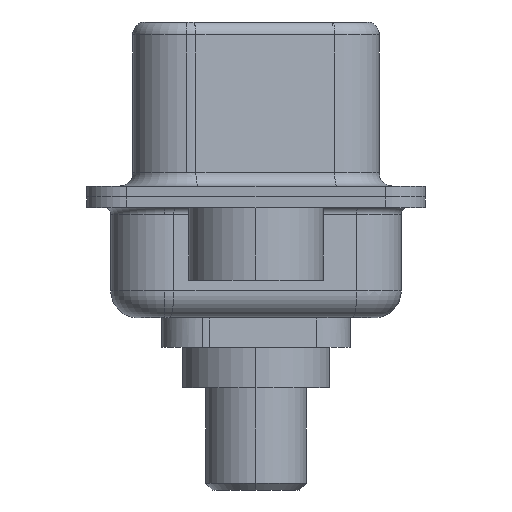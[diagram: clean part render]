
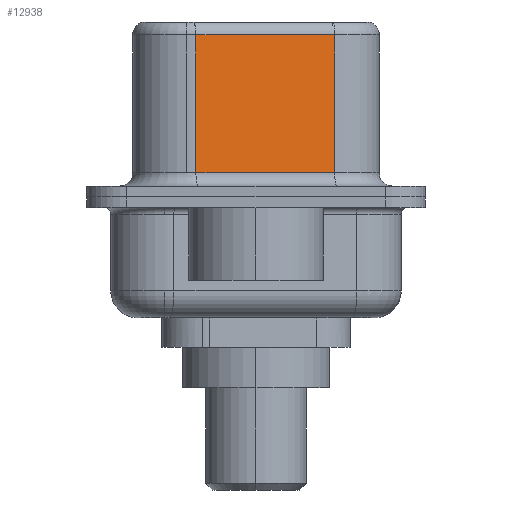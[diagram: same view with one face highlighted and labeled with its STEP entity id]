
A CAD part, left-side view. The second image highlights one B-rep face of the part: STEP entity #12938.
In plain terms, the highlighted planar face has unit normal (-0.985, -0.174, 0).
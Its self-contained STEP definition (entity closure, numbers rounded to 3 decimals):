
#333 = LINE ( 'NONE', #4341, #4810 ) ;
#788 = VECTOR ( 'NONE', #9437, 1000. ) ;
#1344 = CARTESIAN_POINT ( 'NONE',  ( 4.58, -2.927, 6.02 ) ) ;
#3745 = ORIENTED_EDGE ( 'NONE', *, *, #11406, .F. ) ;
#4217 = DIRECTION ( 'NONE',  ( -0.174, 0.985, 0. ) ) ;
#4341 = CARTESIAN_POINT ( 'NONE',  ( 4.58, -2.927, 0.9 ) ) ;
#4394 = DIRECTION ( 'NONE',  ( 0.174, -0.985, 0. ) ) ;
#4810 = VECTOR ( 'NONE', #4394, 1000. ) ;
#5118 = CARTESIAN_POINT ( 'NONE',  ( 3.67, 2.233, 6.02 ) ) ;
#5664 = PLANE ( 'NONE',  #11232 ) ;
#5673 = EDGE_CURVE ( 'NONE', #13320, #16000, #6641, .T. ) ;
#6273 = EDGE_CURVE ( 'NONE', #14563, #13320, #10431, .T. ) ;
#6616 = DIRECTION ( 'NONE',  ( 0., 0., -1. ) ) ;
#6641 = LINE ( 'NONE', #7035, #11606 ) ;
#7016 = DIRECTION ( 'NONE',  ( -0.174, 0.985, 0. ) ) ;
#7035 = CARTESIAN_POINT ( 'NONE',  ( 3.67, 2.233, 6.52 ) ) ;
#7246 = CARTESIAN_POINT ( 'NONE',  ( 4.58, -2.927, 6.52 ) ) ;
#7706 = CARTESIAN_POINT ( 'NONE',  ( 4.58, -2.927, 0.9 ) ) ;
#8736 = ORIENTED_EDGE ( 'NONE', *, *, #6273, .T. ) ;
#8858 = EDGE_CURVE ( 'NONE', #16000, #11761, #333, .T. ) ;
#8911 = VECTOR ( 'NONE', #4217, 1000. ) ;
#9092 = CARTESIAN_POINT ( 'NONE',  ( 4.58, -2.927, 6.02 ) ) ;
#9366 = CARTESIAN_POINT ( 'NONE',  ( 4.58, -2.927, 6.52 ) ) ;
#9437 = DIRECTION ( 'NONE',  ( 0., 0., -1. ) ) ;
#10381 = FACE_OUTER_BOUND ( 'NONE', #14816, .T. ) ;
#10431 = LINE ( 'NONE', #1344, #8911 ) ;
#10659 = ORIENTED_EDGE ( 'NONE', *, *, #5673, .T. ) ;
#11232 = AXIS2_PLACEMENT_3D ( 'NONE', #9366, #14383, #7016 ) ;
#11406 = EDGE_CURVE ( 'NONE', #14563, #11761, #14156, .T. ) ;
#11606 = VECTOR ( 'NONE', #6616, 1000. ) ;
#11761 = VERTEX_POINT ( 'NONE', #7706 ) ;
#12938 = ADVANCED_FACE ( 'NONE', ( #10381 ), #5664, .F. ) ;
#13320 = VERTEX_POINT ( 'NONE', #5118 ) ;
#14129 = ORIENTED_EDGE ( 'NONE', *, *, #8858, .T. ) ;
#14156 = LINE ( 'NONE', #7246, #788 ) ;
#14383 = DIRECTION ( 'NONE',  ( 0.985, 0.174, 0. ) ) ;
#14563 = VERTEX_POINT ( 'NONE', #9092 ) ;
#14816 = EDGE_LOOP ( 'NONE', ( #3745, #8736, #10659, #14129 ) ) ;
#15628 = CARTESIAN_POINT ( 'NONE',  ( 3.67, 2.233, 0.9 ) ) ;
#16000 = VERTEX_POINT ( 'NONE', #15628 ) ;
